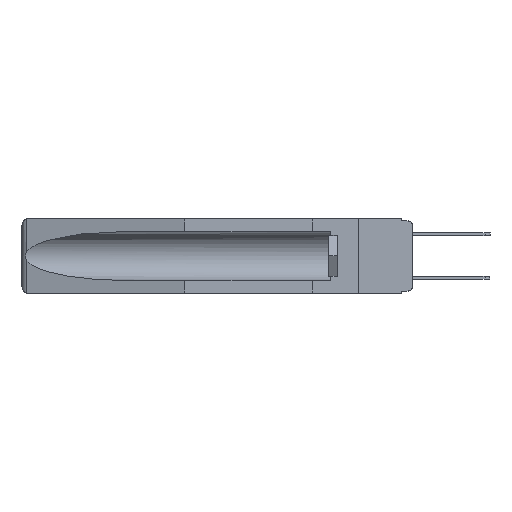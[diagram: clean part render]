
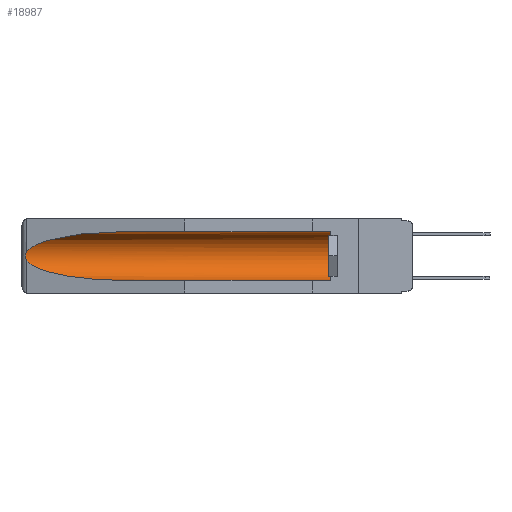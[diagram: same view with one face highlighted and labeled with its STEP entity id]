
A CAD part, left-side view. The second image highlights one B-rep face of the part: STEP entity #18987.
In plain terms, the highlighted cylindrical face has radius 2.857 mm (diameter 5.715 mm), a partial arc.
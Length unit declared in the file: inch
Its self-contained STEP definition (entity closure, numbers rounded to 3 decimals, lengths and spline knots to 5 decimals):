
#843 = VERTEX_POINT ( 'NONE', #8066 ) ;
#1099 = CARTESIAN_POINT ( 'NONE',  ( 0.155, 1.07973, -0.059 ) ) ;
#1363 = VERTEX_POINT ( 'NONE', #9962 ) ;
#1475 = AXIS2_PLACEMENT_3D ( 'NONE', #17504, #4574, #19658 ) ;
#2190 = CARTESIAN_POINT ( 'NONE',  ( 0.2673, 1.5327, -0.16383 ) ) ;
#2657 = CARTESIAN_POINT ( 'NONE',  ( 0.25451, 1.48313, -0.24835 ) ) ;
#3317 = CARTESIAN_POINT ( 'NONE',  ( 0.21114, 1.30732, -0.059 ) ) ;
#3414 = CARTESIAN_POINT ( 'NONE',  ( 0.26537, 1.52718, -0.14972 ) ) ;
#4404 = CARTESIAN_POINT ( 'NONE',  ( 0.2675, 1.53308, -0.17534 ) ) ;
#4501 = CARTESIAN_POINT ( 'NONE',  ( 0.155, -0.30754, -0.059 ) ) ;
#4509 = DIRECTION ( 'NONE',  ( 0., 1., 0. ) ) ;
#4574 = DIRECTION ( 'NONE',  ( 0., -1., 0. ) ) ;
#4862 = CARTESIAN_POINT ( 'NONE',  ( 0.26537, 1.52718, -0.19328 ) ) ;
#6602 = CARTESIAN_POINT ( 'NONE',  ( 0.26655, 1.53094, -0.18657 ) ) ;
#6689 = DIRECTION ( 'NONE',  ( 0., 1., 0. ) ) ;
#7045 = CARTESIAN_POINT ( 'NONE',  ( 0.21114, 1.30732, -0.284 ) ) ;
#7933 = ORIENTED_EDGE ( 'NONE', *, *, #8344, .T. ) ;
#8066 = CARTESIAN_POINT ( 'NONE',  ( 0.155, 0.126, -0.284 ) ) ;
#8344 = EDGE_CURVE ( 'NONE', #1363, #25310, #15117, .T. ) ;
#8634 = VECTOR ( 'NONE', #6689, 39.37008 ) ;
#8761 = CARTESIAN_POINT ( 'NONE',  ( 0.26537, 1.52718, -0.19328 ) ) ;
#9238 = EDGE_CURVE ( 'NONE', #17260, #1363, #9253, .T. ) ;
#9253 =( BOUNDED_CURVE ( )  B_SPLINE_CURVE ( 3, ( #1099, #3317, #16356, #3414 ),
 .UNSPECIFIED., .F., .F. ) 
 B_SPLINE_CURVE_WITH_KNOTS ( ( 4, 4 ),
 ( 4.71239, 6.08839 ),
 .UNSPECIFIED. ) 
 CURVE ( )  GEOMETRIC_REPRESENTATION_ITEM ( )  RATIONAL_B_SPLINE_CURVE ( ( 1., 0.848, 0.848, 1. ) ) 
 REPRESENTATION_ITEM ( '' )  );
#9809 = ORIENTED_EDGE ( 'NONE', *, *, #21482, .T. ) ;
#9962 = CARTESIAN_POINT ( 'NONE',  ( 0.26537, 1.52718, -0.14972 ) ) ;
#10893 = CARTESIAN_POINT ( 'NONE',  ( 0.26537, 1.52718, -0.14972 ) ) ;
#11135 = ORIENTED_EDGE ( 'NONE', *, *, #18120, .T. ) ;
#11267 = EDGE_CURVE ( 'NONE', #25310, #14386, #20309, .T. ) ;
#12748 = VECTOR ( 'NONE', #4509, 39.37008 ) ;
#13065 = CARTESIAN_POINT ( 'NONE',  ( 0.26597, 1.52961, -0.15275 ) ) ;
#13158 = CARTESIAN_POINT ( 'NONE',  ( 0.155, -0.30754, -0.284 ) ) ;
#13824 = CYLINDRICAL_SURFACE ( 'NONE', #23552, 0.1125 ) ;
#13898 = CARTESIAN_POINT ( 'NONE',  ( 0.155, 1.07973, -0.284 ) ) ;
#14386 = VERTEX_POINT ( 'NONE', #13898 ) ;
#15117 = B_SPLINE_CURVE_WITH_KNOTS ( 'NONE', 3,
 ( #10893, #13065, #15208, #2190, #17343, #4404, #19492, #6602, #21644, #8761 ),
 .UNSPECIFIED., .F., .F.,
 ( 4, 2, 2, 2, 4 ),
 ( 0., 0.00029, 0.00058, 0.00087, 0.00117 ),
 .UNSPECIFIED. ) ;
#15208 = CARTESIAN_POINT ( 'NONE',  ( 0.26654, 1.53092, -0.15636 ) ) ;
#16356 = CARTESIAN_POINT ( 'NONE',  ( 0.25451, 1.48313, -0.09465 ) ) ;
#17058 = CARTESIAN_POINT ( 'NONE',  ( 0.26537, 1.52718, -0.19328 ) ) ;
#17207 = EDGE_LOOP ( 'NONE', ( #22638, #7933, #24095, #27705, #11135, #9809 ) ) ;
#17260 = VERTEX_POINT ( 'NONE', #25174 ) ;
#17343 = CARTESIAN_POINT ( 'NONE',  ( 0.2675, 1.53308, -0.16763 ) ) ;
#17504 = CARTESIAN_POINT ( 'NONE',  ( 0.155, 0.126, -0.1715 ) ) ;
#18120 = EDGE_CURVE ( 'NONE', #843, #21544, #18211, .T. ) ;
#18211 = CIRCLE ( 'NONE', #1475, 0.1125 ) ;
#18987 = ADVANCED_FACE ( 'NONE', ( #25796 ), #13824, .F. ) ;
#19079 = LINE ( 'NONE', #13158, #12748 ) ;
#19492 = CARTESIAN_POINT ( 'NONE',  ( 0.2673, 1.53269, -0.17917 ) ) ;
#19658 = DIRECTION ( 'NONE',  ( 0., 0., 1. ) ) ;
#20309 =( BOUNDED_CURVE ( )  B_SPLINE_CURVE ( 3, ( #4862, #2657, #7045, #22085 ),
 .UNSPECIFIED., .F., .F. ) 
 B_SPLINE_CURVE_WITH_KNOTS ( ( 4, 4 ),
 ( 0.1948, 1.5708 ),
 .UNSPECIFIED. ) 
 CURVE ( )  GEOMETRIC_REPRESENTATION_ITEM ( )  RATIONAL_B_SPLINE_CURVE ( ( 1., 0.848, 0.848, 1. ) ) 
 REPRESENTATION_ITEM ( '' )  );
#20933 = DIRECTION ( 'NONE',  ( 0., 0., 1. ) ) ;
#21482 = EDGE_CURVE ( 'NONE', #21544, #17260, #25730, .T. ) ;
#21544 = VERTEX_POINT ( 'NONE', #23965 ) ;
#21644 = CARTESIAN_POINT ( 'NONE',  ( 0.26597, 1.5296, -0.19026 ) ) ;
#22085 = CARTESIAN_POINT ( 'NONE',  ( 0.155, 1.07973, -0.284 ) ) ;
#22638 = ORIENTED_EDGE ( 'NONE', *, *, #9238, .T. ) ;
#23552 = AXIS2_PLACEMENT_3D ( 'NONE', #25197, #27296, #20933 ) ;
#23965 = CARTESIAN_POINT ( 'NONE',  ( 0.155, 0.126, -0.059 ) ) ;
#24095 = ORIENTED_EDGE ( 'NONE', *, *, #11267, .T. ) ;
#25174 = CARTESIAN_POINT ( 'NONE',  ( 0.155, 1.07973, -0.059 ) ) ;
#25197 = CARTESIAN_POINT ( 'NONE',  ( 0.155, -0.30754, -0.1715 ) ) ;
#25310 = VERTEX_POINT ( 'NONE', #17058 ) ;
#25730 = LINE ( 'NONE', #4501, #8634 ) ;
#25796 = FACE_OUTER_BOUND ( 'NONE', #17207, .T. ) ;
#27296 = DIRECTION ( 'NONE',  ( 0., 1., 0. ) ) ;
#27705 = ORIENTED_EDGE ( 'NONE', *, *, #27830, .F. ) ;
#27830 = EDGE_CURVE ( 'NONE', #843, #14386, #19079, .T. ) ;
